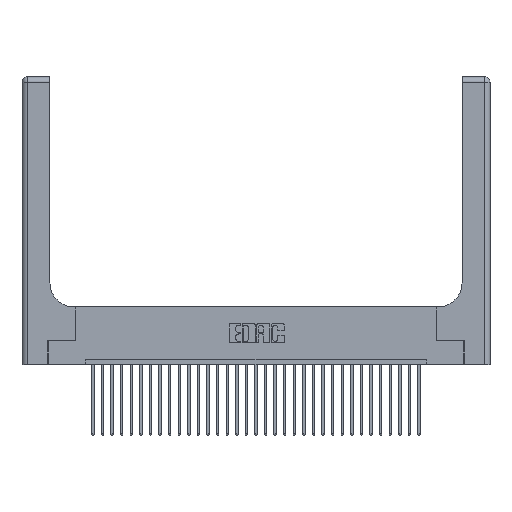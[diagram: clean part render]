
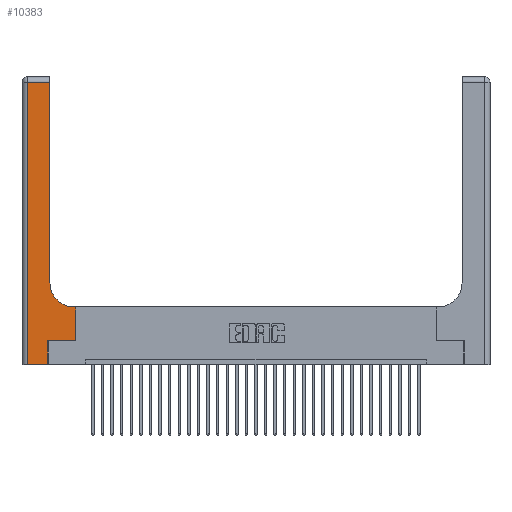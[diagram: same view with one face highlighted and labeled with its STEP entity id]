
A CAD part, top view. The second image highlights one B-rep face of the part: STEP entity #10383.
In plain terms, the highlighted planar face has unit normal (0, 0, 1).
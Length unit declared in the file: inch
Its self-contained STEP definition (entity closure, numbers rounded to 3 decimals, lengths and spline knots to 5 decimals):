
#67 = VERTEX_POINT ( 'NONE', #7631 ) ;
#190 = VECTOR ( 'NONE', #11504, 39.37008 ) ;
#745 = DIRECTION ( 'NONE',  ( -1., 0., 0. ) ) ;
#807 = CARTESIAN_POINT ( 'NONE',  ( 0.2915, 3., 0.37 ) ) ;
#1052 = CARTESIAN_POINT ( 'NONE',  ( 0.269, 0.25, 0.37 ) ) ;
#1639 = CARTESIAN_POINT ( 'NONE',  ( 0.2915, 0.6, 0.37 ) ) ;
#1857 = VECTOR ( 'NONE', #3518, 39.37008 ) ;
#2078 = ORIENTED_EDGE ( 'NONE', *, *, #20569, .T. ) ;
#2915 = DIRECTION ( 'NONE',  ( 0., 0., -1. ) ) ;
#3518 = DIRECTION ( 'NONE',  ( 0., 1., 0. ) ) ;
#3826 = CIRCLE ( 'NONE', #26199, 0.25 ) ;
#4072 = LINE ( 'NONE', #26532, #190 ) ;
#4302 = CARTESIAN_POINT ( 'NONE',  ( 0.5585, 0.6, 0.37 ) ) ;
#4464 = VECTOR ( 'NONE', #7229, 39.37008 ) ;
#5050 = EDGE_LOOP ( 'NONE', ( #27912, #5067, #30651, #5692, #16971, #13847, #30541, #30124, #2078 ) ) ;
#5067 = ORIENTED_EDGE ( 'NONE', *, *, #25658, .T. ) ;
#5692 = ORIENTED_EDGE ( 'NONE', *, *, #25664, .T. ) ;
#5716 = VECTOR ( 'NONE', #16555, 39.37008 ) ;
#6079 = VECTOR ( 'NONE', #8530, 39.37008 ) ;
#6457 = EDGE_CURVE ( 'NONE', #17195, #7278, #21838, .T. ) ;
#7229 = DIRECTION ( 'NONE',  ( 0., 1., 0. ) ) ;
#7278 = VERTEX_POINT ( 'NONE', #16868 ) ;
#7295 = VERTEX_POINT ( 'NONE', #19280 ) ;
#7631 = CARTESIAN_POINT ( 'NONE',  ( 0.5415, 0.6, 0.37 ) ) ;
#8177 = CARTESIAN_POINT ( 'NONE',  ( 0.5415, 0.85, 0.37 ) ) ;
#8530 = DIRECTION ( 'NONE',  ( -1., 0., 0. ) ) ;
#8661 = DIRECTION ( 'NONE',  ( 0., 0., -1. ) ) ;
#9606 = LINE ( 'NONE', #1639, #6079 ) ;
#9640 = CARTESIAN_POINT ( 'NONE',  ( 0.5585, 0.25, 0.37 ) ) ;
#10011 = CARTESIAN_POINT ( 'NONE',  ( 0.2915, 2.94, 0.37 ) ) ;
#10383 = ADVANCED_FACE ( 'NONE', ( #28705 ), #29126, .F. ) ;
#10536 = VERTEX_POINT ( 'NONE', #25173 ) ;
#11234 = CARTESIAN_POINT ( 'NONE',  ( 0., 3., 0.37 ) ) ;
#11409 = VERTEX_POINT ( 'NONE', #9640 ) ;
#11504 = DIRECTION ( 'NONE',  ( 1., 0., 0. ) ) ;
#11888 = DIRECTION ( 'NONE',  ( 0., -1., 0. ) ) ;
#11889 = AXIS2_PLACEMENT_3D ( 'NONE', #11234, #8661, #745 ) ;
#12077 = LINE ( 'NONE', #807, #1857 ) ;
#13690 = EDGE_CURVE ( 'NONE', #7295, #30552, #12077, .T. ) ;
#13847 = ORIENTED_EDGE ( 'NONE', *, *, #26084, .T. ) ;
#15142 = VECTOR ( 'NONE', #20985, 39.37008 ) ;
#15210 = VERTEX_POINT ( 'NONE', #27284 ) ;
#16555 = DIRECTION ( 'NONE',  ( -1., 0., 0. ) ) ;
#16868 = CARTESIAN_POINT ( 'NONE',  ( 0.269, 0.25, 0.37 ) ) ;
#16971 = ORIENTED_EDGE ( 'NONE', *, *, #6457, .T. ) ;
#17021 = LINE ( 'NONE', #22260, #4464 ) ;
#17195 = VERTEX_POINT ( 'NONE', #17552 ) ;
#17552 = CARTESIAN_POINT ( 'NONE',  ( 0.269, 0., 0.37 ) ) ;
#19280 = CARTESIAN_POINT ( 'NONE',  ( 0.2915, 0.85, 0.37 ) ) ;
#19586 = VERTEX_POINT ( 'NONE', #4302 ) ;
#19597 = EDGE_CURVE ( 'NONE', #10536, #15210, #21853, .T. ) ;
#20569 = EDGE_CURVE ( 'NONE', #67, #7295, #3826, .T. ) ;
#20985 = DIRECTION ( 'NONE',  ( 0., 1., 0. ) ) ;
#21400 = CARTESIAN_POINT ( 'NONE',  ( 0., 2.94, 0.37 ) ) ;
#21838 = LINE ( 'NONE', #23166, #15142 ) ;
#21853 = LINE ( 'NONE', #27107, #23404 ) ;
#22139 = VECTOR ( 'NONE', #28687, 39.37008 ) ;
#22260 = CARTESIAN_POINT ( 'NONE',  ( 0.5585, 0.25, 0.37 ) ) ;
#23166 = CARTESIAN_POINT ( 'NONE',  ( 0.269, 0., 0.37 ) ) ;
#23404 = VECTOR ( 'NONE', #11888, 39.37008 ) ;
#25173 = CARTESIAN_POINT ( 'NONE',  ( 0.06, 2.94, 0.37 ) ) ;
#25658 = EDGE_CURVE ( 'NONE', #30552, #10536, #28831, .T. ) ;
#25664 = EDGE_CURVE ( 'NONE', #15210, #17195, #4072, .T. ) ;
#25996 = EDGE_CURVE ( 'NONE', #11409, #19586, #17021, .T. ) ;
#26084 = EDGE_CURVE ( 'NONE', #7278, #11409, #28768, .T. ) ;
#26199 = AXIS2_PLACEMENT_3D ( 'NONE', #8177, #2915, #30669 ) ;
#26532 = CARTESIAN_POINT ( 'NONE',  ( 0., 0., 0.37 ) ) ;
#27107 = CARTESIAN_POINT ( 'NONE',  ( 0.06, 3., 0.37 ) ) ;
#27284 = CARTESIAN_POINT ( 'NONE',  ( 0.06, 0., 0.37 ) ) ;
#27912 = ORIENTED_EDGE ( 'NONE', *, *, #13690, .T. ) ;
#28687 = DIRECTION ( 'NONE',  ( 1., 0., 0. ) ) ;
#28705 = FACE_OUTER_BOUND ( 'NONE', #5050, .T. ) ;
#28768 = LINE ( 'NONE', #1052, #22139 ) ;
#28831 = LINE ( 'NONE', #21400, #5716 ) ;
#29126 = PLANE ( 'NONE',  #11889 ) ;
#30124 = ORIENTED_EDGE ( 'NONE', *, *, #30874, .T. ) ;
#30541 = ORIENTED_EDGE ( 'NONE', *, *, #25996, .T. ) ;
#30552 = VERTEX_POINT ( 'NONE', #10011 ) ;
#30651 = ORIENTED_EDGE ( 'NONE', *, *, #19597, .T. ) ;
#30669 = DIRECTION ( 'NONE',  ( 1., 0., 0. ) ) ;
#30874 = EDGE_CURVE ( 'NONE', #19586, #67, #9606, .T. ) ;
